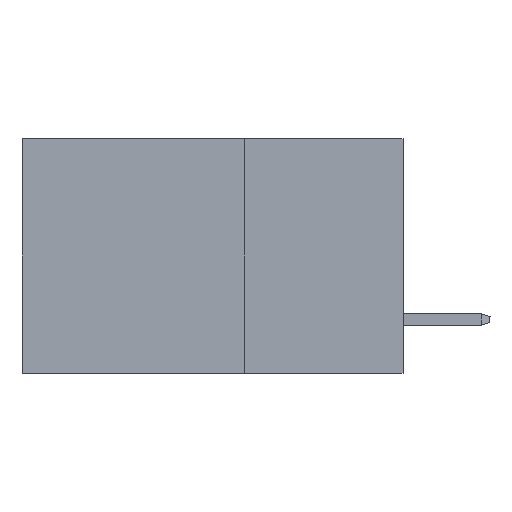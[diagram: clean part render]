
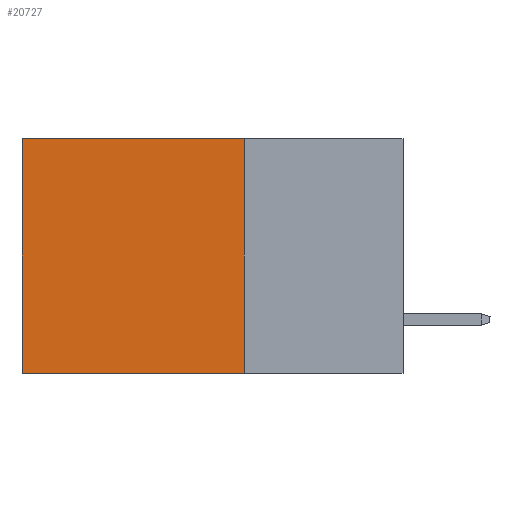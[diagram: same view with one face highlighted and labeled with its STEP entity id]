
A CAD part, left-side view. The second image highlights one B-rep face of the part: STEP entity #20727.
In plain terms, the highlighted planar face has unit normal (-1, 0, 0).
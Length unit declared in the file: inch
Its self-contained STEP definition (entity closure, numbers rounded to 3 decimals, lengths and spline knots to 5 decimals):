
#997 = ORIENTED_EDGE ( 'NONE', *, *, #27683, .T. ) ;
#1099 = EDGE_CURVE ( 'NONE', #16036, #12839, #12027, .T. ) ;
#2614 = EDGE_CURVE ( 'NONE', #8476, #16036, #7547, .T. ) ;
#3707 = LINE ( 'NONE', #8519, #20310 ) ;
#5525 = DIRECTION ( 'NONE',  ( 0., 0., -1. ) ) ;
#7532 = EDGE_LOOP ( 'NONE', ( #23229, #33840, #17614, #997 ) ) ;
#7547 = LINE ( 'NONE', #30183, #8766 ) ;
#8476 = VERTEX_POINT ( 'NONE', #25546 ) ;
#8519 = CARTESIAN_POINT ( 'NONE',  ( 0.2875, 0.25, 0. ) ) ;
#8766 = VECTOR ( 'NONE', #5525, 39.37008 ) ;
#10239 = LINE ( 'NONE', #29924, #24113 ) ;
#11463 = DIRECTION ( 'NONE',  ( 0., 1., 0. ) ) ;
#11931 = CARTESIAN_POINT ( 'NONE',  ( 0.2875, 0.25, 0. ) ) ;
#12027 = LINE ( 'NONE', #31531, #22975 ) ;
#12122 = DIRECTION ( 'NONE',  ( 0., 0., -1. ) ) ;
#12839 = VERTEX_POINT ( 'NONE', #32960 ) ;
#13326 = AXIS2_PLACEMENT_3D ( 'NONE', #11931, #26237, #12122 ) ;
#16036 = VERTEX_POINT ( 'NONE', #35647 ) ;
#17614 = ORIENTED_EDGE ( 'NONE', *, *, #2614, .F. ) ;
#18725 = CARTESIAN_POINT ( 'NONE',  ( 0.2875, 0.6, 0. ) ) ;
#20310 = VECTOR ( 'NONE', #22864, 39.37008 ) ;
#20727 = ADVANCED_FACE ( 'NONE', ( #34572 ), #29355, .F. ) ;
#22864 = DIRECTION ( 'NONE',  ( 0., 1., 0. ) ) ;
#22975 = VECTOR ( 'NONE', #11463, 39.37008 ) ;
#23229 = ORIENTED_EDGE ( 'NONE', *, *, #31758, .T. ) ;
#24113 = VECTOR ( 'NONE', #32394, 39.37008 ) ;
#25546 = CARTESIAN_POINT ( 'NONE',  ( 0.2875, 0.25, 0. ) ) ;
#26237 = DIRECTION ( 'NONE',  ( 1., 0., 0. ) ) ;
#27683 = EDGE_CURVE ( 'NONE', #8476, #30846, #3707, .T. ) ;
#29355 = PLANE ( 'NONE',  #13326 ) ;
#29924 = CARTESIAN_POINT ( 'NONE',  ( 0.2875, 0.6, 0. ) ) ;
#30183 = CARTESIAN_POINT ( 'NONE',  ( 0.2875, 0.25, 0. ) ) ;
#30846 = VERTEX_POINT ( 'NONE', #18725 ) ;
#31531 = CARTESIAN_POINT ( 'NONE',  ( 0.2875, 0.25, -0.37 ) ) ;
#31758 = EDGE_CURVE ( 'NONE', #30846, #12839, #10239, .T. ) ;
#32394 = DIRECTION ( 'NONE',  ( 0., 0., -1. ) ) ;
#32960 = CARTESIAN_POINT ( 'NONE',  ( 0.2875, 0.6, -0.37 ) ) ;
#33840 = ORIENTED_EDGE ( 'NONE', *, *, #1099, .F. ) ;
#34572 = FACE_OUTER_BOUND ( 'NONE', #7532, .T. ) ;
#35647 = CARTESIAN_POINT ( 'NONE',  ( 0.2875, 0.25, -0.37 ) ) ;
